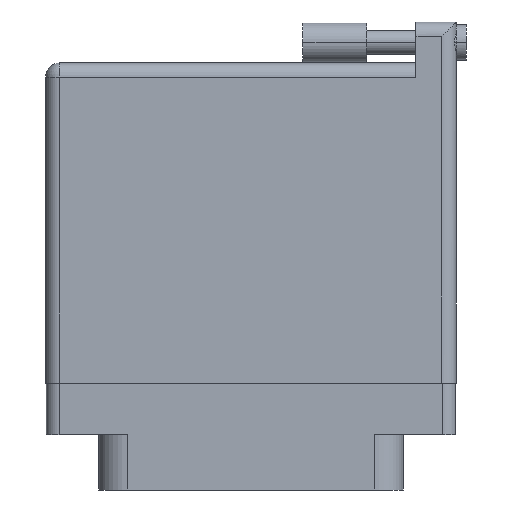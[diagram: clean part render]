
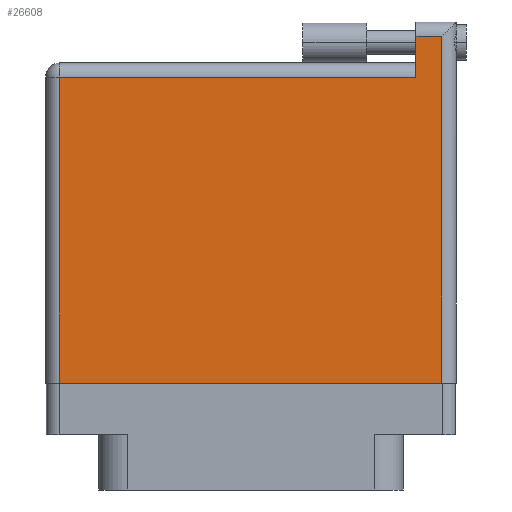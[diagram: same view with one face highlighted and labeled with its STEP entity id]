
A CAD part, front view. The second image highlights one B-rep face of the part: STEP entity #26608.
In plain terms, the highlighted face is planar.
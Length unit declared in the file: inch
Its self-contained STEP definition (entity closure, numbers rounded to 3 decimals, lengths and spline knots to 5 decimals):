
#105 = DIRECTION ( 'NONE',  ( 0., -1., 0. ) ) ;
#224 = DIRECTION ( 'NONE',  ( 0., 0., -1. ) ) ;
#2767 = CARTESIAN_POINT ( 'NONE',  ( -1.004, 1.466, 0.4495 ) ) ;
#2904 = LINE ( 'NONE', #32097, #21997 ) ;
#4651 = VERTEX_POINT ( 'NONE', #17790 ) ;
#5244 = VECTOR ( 'NONE', #32444, 39.37008 ) ;
#5614 = EDGE_LOOP ( 'NONE', ( #10658, #35412, #8681, #18222, #24588, #10882 ) ) ;
#7272 = CARTESIAN_POINT ( 'NONE',  ( -1.004, 1.396, 0.4495 ) ) ;
#8176 = CARTESIAN_POINT ( 'NONE',  ( -1.004, 1.596, 0.4495 ) ) ;
#8383 = CARTESIAN_POINT ( 'NONE',  ( 0.807, 1.596, 0.4495 ) ) ;
#8681 = ORIENTED_EDGE ( 'NONE', *, *, #13598, .T. ) ;
#8773 = FACE_OUTER_BOUND ( 'NONE', #5614, .T. ) ;
#9761 = VERTEX_POINT ( 'NONE', #8383 ) ;
#9765 = LINE ( 'NONE', #31175, #10635 ) ;
#10635 = VECTOR ( 'NONE', #20205, 39.37008 ) ;
#10658 = ORIENTED_EDGE ( 'NONE', *, *, #14743, .T. ) ;
#10882 = ORIENTED_EDGE ( 'NONE', *, *, #20110, .T. ) ;
#11616 = VERTEX_POINT ( 'NONE', #21012 ) ;
#11854 = EDGE_CURVE ( 'NONE', #28113, #11616, #26480, .T. ) ;
#12904 = CARTESIAN_POINT ( 'NONE',  ( 0.934, -0.1, 0.4495 ) ) ;
#13457 = CARTESIAN_POINT ( 'NONE',  ( 0.934, 1.666, 0.4495 ) ) ;
#13598 = EDGE_CURVE ( 'NONE', #11616, #9761, #28968, .T. ) ;
#14008 = CARTESIAN_POINT ( 'NONE',  ( 0.807, 1.666, 0.4495 ) ) ;
#14743 = EDGE_CURVE ( 'NONE', #23862, #28113, #2904, .T. ) ;
#15264 = VERTEX_POINT ( 'NONE', #32997 ) ;
#16136 = VECTOR ( 'NONE', #105, 39.37008 ) ;
#17790 = CARTESIAN_POINT ( 'NONE',  ( 0.807, 1.396, 0.4495 ) ) ;
#18222 = ORIENTED_EDGE ( 'NONE', *, *, #26591, .T. ) ;
#19709 = EDGE_CURVE ( 'NONE', #4651, #15264, #21077, .T. ) ;
#20110 = EDGE_CURVE ( 'NONE', #15264, #23862, #9765, .T. ) ;
#20205 = DIRECTION ( 'NONE',  ( 0., -1., 0. ) ) ;
#21012 = CARTESIAN_POINT ( 'NONE',  ( 0.934, 1.596, 0.4495 ) ) ;
#21077 = LINE ( 'NONE', #7272, #21517 ) ;
#21517 = VECTOR ( 'NONE', #21532, 39.37008 ) ;
#21532 = DIRECTION ( 'NONE',  ( -1., 0., 0. ) ) ;
#21997 = VECTOR ( 'NONE', #26564, 39.37008 ) ;
#23771 = VECTOR ( 'NONE', #33176, 39.37008 ) ;
#23862 = VERTEX_POINT ( 'NONE', #30472 ) ;
#24588 = ORIENTED_EDGE ( 'NONE', *, *, #19709, .T. ) ;
#26480 = LINE ( 'NONE', #13457, #5244 ) ;
#26564 = DIRECTION ( 'NONE',  ( 1., 0., 0. ) ) ;
#26591 = EDGE_CURVE ( 'NONE', #9761, #4651, #33851, .T. ) ;
#26608 = ADVANCED_FACE ( 'NONE', ( #8773 ), #27686, .F. ) ;
#27686 = PLANE ( 'NONE',  #34426 ) ;
#28113 = VERTEX_POINT ( 'NONE', #12904 ) ;
#28968 = LINE ( 'NONE', #8176, #23771 ) ;
#30366 = DIRECTION ( 'NONE',  ( -1., 0., 0. ) ) ;
#30472 = CARTESIAN_POINT ( 'NONE',  ( -0.934, -0.1, 0.4495 ) ) ;
#31175 = CARTESIAN_POINT ( 'NONE',  ( -0.934, -0.1, 0.4495 ) ) ;
#32097 = CARTESIAN_POINT ( 'NONE',  ( -1.004, -0.1, 0.4495 ) ) ;
#32444 = DIRECTION ( 'NONE',  ( 0., 1., 0. ) ) ;
#32997 = CARTESIAN_POINT ( 'NONE',  ( -0.934, 1.396, 0.4495 ) ) ;
#33176 = DIRECTION ( 'NONE',  ( -1., 0., 0. ) ) ;
#33851 = LINE ( 'NONE', #14008, #16136 ) ;
#34426 = AXIS2_PLACEMENT_3D ( 'NONE', #2767, #224, #30366 ) ;
#35412 = ORIENTED_EDGE ( 'NONE', *, *, #11854, .T. ) ;
